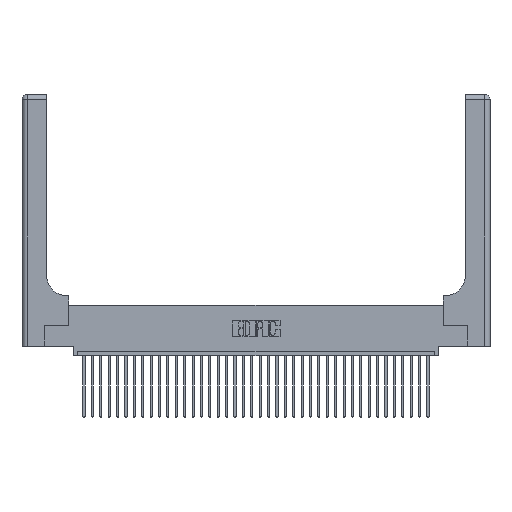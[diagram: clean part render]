
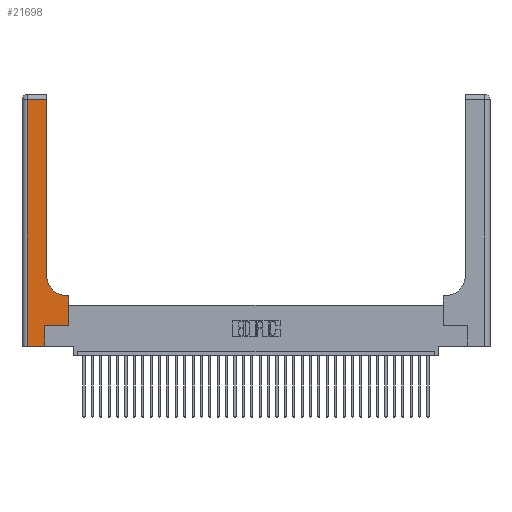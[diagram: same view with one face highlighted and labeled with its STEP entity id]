
A CAD part, top view. The second image highlights one B-rep face of the part: STEP entity #21698.
In plain terms, the highlighted planar face has unit normal (0, 0, 1).
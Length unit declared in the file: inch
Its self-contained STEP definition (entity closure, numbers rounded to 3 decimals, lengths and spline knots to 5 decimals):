
#854 = DIRECTION ( 'NONE',  ( 0., -1., 0. ) ) ;
#1109 = CARTESIAN_POINT ( 'NONE',  ( 0.5415, 0.85, 0.37 ) ) ;
#1149 = VECTOR ( 'NONE', #30459, 39.37008 ) ;
#2270 = DIRECTION ( 'NONE',  ( 0., 0., -1. ) ) ;
#2587 = EDGE_CURVE ( 'NONE', #29290, #8610, #32436, .T. ) ;
#3929 = EDGE_CURVE ( 'NONE', #25081, #29290, #15492, .T. ) ;
#3950 = CARTESIAN_POINT ( 'NONE',  ( 0., 0., 0.37 ) ) ;
#4339 = DIRECTION ( 'NONE',  ( 0., 0., -1. ) ) ;
#4647 = DIRECTION ( 'NONE',  ( 0., 1., 0. ) ) ;
#4726 = VECTOR ( 'NONE', #25185, 39.37008 ) ;
#4979 = VERTEX_POINT ( 'NONE', #8253 ) ;
#5418 = DIRECTION ( 'NONE',  ( -1., 0., 0. ) ) ;
#6033 = LINE ( 'NONE', #30286, #10511 ) ;
#6367 = EDGE_LOOP ( 'NONE', ( #18508, #24651, #22709, #27206, #8500, #36593, #8973, #13245, #9505 ) ) ;
#6404 = CARTESIAN_POINT ( 'NONE',  ( 0.269, 0., 0.37 ) ) ;
#6981 = LINE ( 'NONE', #19155, #1149 ) ;
#7499 = VERTEX_POINT ( 'NONE', #34893 ) ;
#7864 = LINE ( 'NONE', #27799, #4726 ) ;
#7904 = CARTESIAN_POINT ( 'NONE',  ( 0.06, 2.94, 0.37 ) ) ;
#8076 = VERTEX_POINT ( 'NONE', #26311 ) ;
#8253 = CARTESIAN_POINT ( 'NONE',  ( 0.5585, 0.6, 0.37 ) ) ;
#8394 = CARTESIAN_POINT ( 'NONE',  ( 0.2915, 0.6, 0.37 ) ) ;
#8500 = ORIENTED_EDGE ( 'NONE', *, *, #32062, .T. ) ;
#8610 = VERTEX_POINT ( 'NONE', #6404 ) ;
#8911 = CARTESIAN_POINT ( 'NONE',  ( 0.2915, 2.94, 0.37 ) ) ;
#8973 = ORIENTED_EDGE ( 'NONE', *, *, #35143, .T. ) ;
#9505 = ORIENTED_EDGE ( 'NONE', *, *, #34303, .T. ) ;
#9523 = LINE ( 'NONE', #11028, #11680 ) ;
#10081 = VERTEX_POINT ( 'NONE', #8911 ) ;
#10215 = DIRECTION ( 'NONE',  ( 1., 0., 0. ) ) ;
#10511 = VECTOR ( 'NONE', #4647, 39.37008 ) ;
#11028 = CARTESIAN_POINT ( 'NONE',  ( 0.269, 0., 0.37 ) ) ;
#11415 = EDGE_CURVE ( 'NONE', #32108, #12553, #6981, .T. ) ;
#11680 = VECTOR ( 'NONE', #24722, 39.37008 ) ;
#12553 = VERTEX_POINT ( 'NONE', #16299 ) ;
#12919 = AXIS2_PLACEMENT_3D ( 'NONE', #36381, #2270, #19363 ) ;
#12974 = AXIS2_PLACEMENT_3D ( 'NONE', #1109, #4339, #21030 ) ;
#13245 = ORIENTED_EDGE ( 'NONE', *, *, #23099, .T. ) ;
#14481 = VECTOR ( 'NONE', #34456, 39.37008 ) ;
#15492 = LINE ( 'NONE', #34595, #33713 ) ;
#16299 = CARTESIAN_POINT ( 'NONE',  ( 0.5585, 0.25, 0.37 ) ) ;
#18286 = CIRCLE ( 'NONE', #12974, 0.25 ) ;
#18508 = ORIENTED_EDGE ( 'NONE', *, *, #30768, .T. ) ;
#18712 = CARTESIAN_POINT ( 'NONE',  ( 0.06, 0., 0.37 ) ) ;
#19155 = CARTESIAN_POINT ( 'NONE',  ( 0.269, 0.25, 0.37 ) ) ;
#19363 = DIRECTION ( 'NONE',  ( -1., 0., 0. ) ) ;
#20161 = LINE ( 'NONE', #28435, #31291 ) ;
#21030 = DIRECTION ( 'NONE',  ( 1., 0., 0. ) ) ;
#21698 = ADVANCED_FACE ( 'NONE', ( #34006 ), #33880, .F. ) ;
#22709 = ORIENTED_EDGE ( 'NONE', *, *, #3929, .T. ) ;
#23099 = EDGE_CURVE ( 'NONE', #4979, #8076, #24280, .T. ) ;
#24280 = LINE ( 'NONE', #8394, #14481 ) ;
#24651 = ORIENTED_EDGE ( 'NONE', *, *, #32210, .T. ) ;
#24722 = DIRECTION ( 'NONE',  ( 0., 1., 0. ) ) ;
#25081 = VERTEX_POINT ( 'NONE', #7904 ) ;
#25185 = DIRECTION ( 'NONE',  ( 0., 1., 0. ) ) ;
#25308 = VECTOR ( 'NONE', #10215, 39.37008 ) ;
#26311 = CARTESIAN_POINT ( 'NONE',  ( 0.5415, 0.6, 0.37 ) ) ;
#27206 = ORIENTED_EDGE ( 'NONE', *, *, #2587, .T. ) ;
#27799 = CARTESIAN_POINT ( 'NONE',  ( 0.5585, 0.25, 0.37 ) ) ;
#28435 = CARTESIAN_POINT ( 'NONE',  ( 0., 2.94, 0.37 ) ) ;
#29290 = VERTEX_POINT ( 'NONE', #18712 ) ;
#30286 = CARTESIAN_POINT ( 'NONE',  ( 0.2915, 3., 0.37 ) ) ;
#30459 = DIRECTION ( 'NONE',  ( 1., 0., 0. ) ) ;
#30768 = EDGE_CURVE ( 'NONE', #7499, #10081, #6033, .T. ) ;
#30928 = CARTESIAN_POINT ( 'NONE',  ( 0.269, 0.25, 0.37 ) ) ;
#31291 = VECTOR ( 'NONE', #5418, 39.37008 ) ;
#32062 = EDGE_CURVE ( 'NONE', #8610, #32108, #9523, .T. ) ;
#32108 = VERTEX_POINT ( 'NONE', #30928 ) ;
#32210 = EDGE_CURVE ( 'NONE', #10081, #25081, #20161, .T. ) ;
#32436 = LINE ( 'NONE', #3950, #25308 ) ;
#33713 = VECTOR ( 'NONE', #854, 39.37008 ) ;
#33880 = PLANE ( 'NONE',  #12919 ) ;
#34006 = FACE_OUTER_BOUND ( 'NONE', #6367, .T. ) ;
#34303 = EDGE_CURVE ( 'NONE', #8076, #7499, #18286, .T. ) ;
#34456 = DIRECTION ( 'NONE',  ( -1., 0., 0. ) ) ;
#34595 = CARTESIAN_POINT ( 'NONE',  ( 0.06, 3., 0.37 ) ) ;
#34893 = CARTESIAN_POINT ( 'NONE',  ( 0.2915, 0.85, 0.37 ) ) ;
#35143 = EDGE_CURVE ( 'NONE', #12553, #4979, #7864, .T. ) ;
#36381 = CARTESIAN_POINT ( 'NONE',  ( 0., 3., 0.37 ) ) ;
#36593 = ORIENTED_EDGE ( 'NONE', *, *, #11415, .T. ) ;
